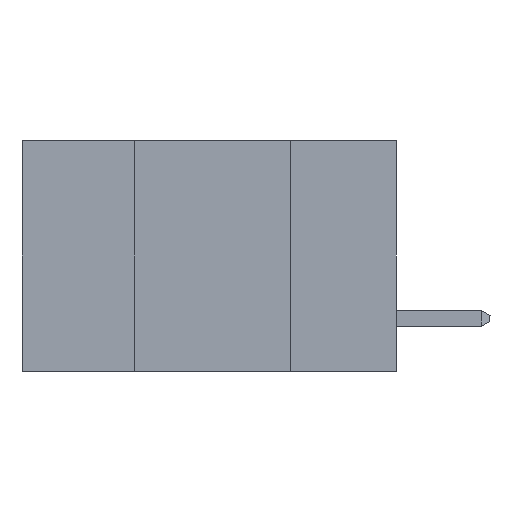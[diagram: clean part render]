
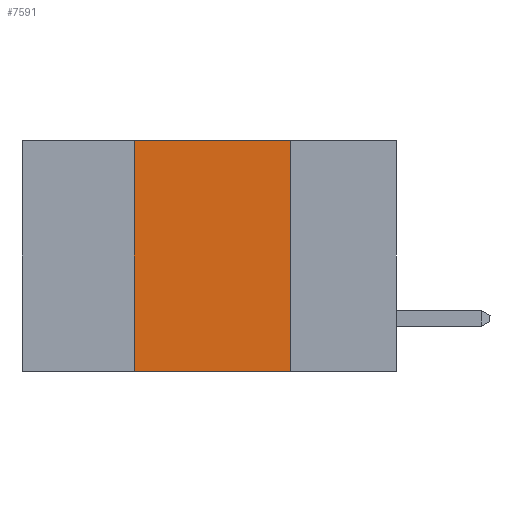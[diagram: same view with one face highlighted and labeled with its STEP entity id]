
A CAD part, left-side view. The second image highlights one B-rep face of the part: STEP entity #7591.
In plain terms, the highlighted planar face has unit normal (-1, 0, 0).
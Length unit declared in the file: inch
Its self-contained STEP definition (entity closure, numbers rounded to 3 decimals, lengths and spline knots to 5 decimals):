
#322 = EDGE_CURVE ( 'NONE', #6241, #5961, #6436, .T. ) ;
#361 = ORIENTED_EDGE ( 'NONE', *, *, #1670, .F. ) ;
#794 = PLANE ( 'NONE',  #2249 ) ;
#799 = DIRECTION ( 'NONE',  ( 0., -1., 0. ) ) ;
#1670 = EDGE_CURVE ( 'NONE', #5961, #7390, #5812, .T. ) ;
#2249 = AXIS2_PLACEMENT_3D ( 'NONE', #11305, #6551, #4461 ) ;
#2398 = EDGE_LOOP ( 'NONE', ( #361, #11049, #4555, #12029 ) ) ;
#2826 = VECTOR ( 'NONE', #11013, 39.37008 ) ;
#3187 = CARTESIAN_POINT ( 'NONE',  ( 0., 0.6, -0.37 ) ) ;
#3965 = DIRECTION ( 'NONE',  ( 0., 0., -1. ) ) ;
#4461 = DIRECTION ( 'NONE',  ( 0., 0., -1. ) ) ;
#4555 = ORIENTED_EDGE ( 'NONE', *, *, #5348, .F. ) ;
#4945 = CARTESIAN_POINT ( 'NONE',  ( 0., 0.17, 0. ) ) ;
#5348 = EDGE_CURVE ( 'NONE', #8818, #6241, #8133, .T. ) ;
#5812 = LINE ( 'NONE', #5992, #11215 ) ;
#5961 = VERTEX_POINT ( 'NONE', #4945 ) ;
#5992 = CARTESIAN_POINT ( 'NONE',  ( 0., 0.17, -0.37 ) ) ;
#6126 = CARTESIAN_POINT ( 'NONE',  ( 0., 0.17, -0.37 ) ) ;
#6155 = DIRECTION ( 'NONE',  ( 0., -1., 0. ) ) ;
#6241 = VERTEX_POINT ( 'NONE', #12016 ) ;
#6436 = LINE ( 'NONE', #10262, #9246 ) ;
#6551 = DIRECTION ( 'NONE',  ( 1., 0., 0. ) ) ;
#6686 = VECTOR ( 'NONE', #6155, 39.37008 ) ;
#7179 = CARTESIAN_POINT ( 'NONE',  ( 0., 0.42, -0.37 ) ) ;
#7390 = VERTEX_POINT ( 'NONE', #6126 ) ;
#7591 = ADVANCED_FACE ( 'NONE', ( #12224 ), #794, .F. ) ;
#8133 = LINE ( 'NONE', #7179, #2826 ) ;
#8818 = VERTEX_POINT ( 'NONE', #12161 ) ;
#9246 = VECTOR ( 'NONE', #799, 39.37008 ) ;
#10262 = CARTESIAN_POINT ( 'NONE',  ( 0., 0.6, 0. ) ) ;
#10850 = LINE ( 'NONE', #3187, #6686 ) ;
#10860 = EDGE_CURVE ( 'NONE', #8818, #7390, #10850, .T. ) ;
#11013 = DIRECTION ( 'NONE',  ( 0., 0., 1. ) ) ;
#11049 = ORIENTED_EDGE ( 'NONE', *, *, #322, .F. ) ;
#11215 = VECTOR ( 'NONE', #3965, 39.37008 ) ;
#11305 = CARTESIAN_POINT ( 'NONE',  ( 0., 0.6, 0. ) ) ;
#12016 = CARTESIAN_POINT ( 'NONE',  ( 0., 0.42, 0. ) ) ;
#12029 = ORIENTED_EDGE ( 'NONE', *, *, #10860, .T. ) ;
#12161 = CARTESIAN_POINT ( 'NONE',  ( 0., 0.42, -0.37 ) ) ;
#12224 = FACE_OUTER_BOUND ( 'NONE', #2398, .T. ) ;
